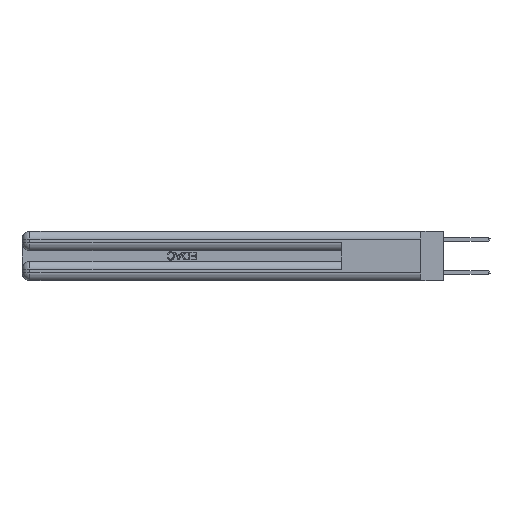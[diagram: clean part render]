
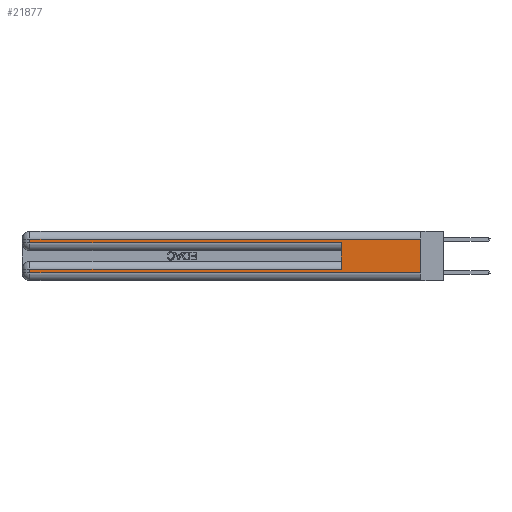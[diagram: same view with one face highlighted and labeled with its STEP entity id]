
A CAD part, left-side view. The second image highlights one B-rep face of the part: STEP entity #21877.
In plain terms, the highlighted planar face has unit normal (-1, 0, 0).
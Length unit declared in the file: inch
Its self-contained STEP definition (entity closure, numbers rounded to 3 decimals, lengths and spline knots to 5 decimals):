
#136 = PLANE ( 'NONE',  #1682 ) ;
#497 = DIRECTION ( 'NONE',  ( 0., -1., 0. ) ) ;
#635 = DIRECTION ( 'NONE',  ( 0., 0., -1. ) ) ;
#665 = VECTOR ( 'NONE', #23990, 39.37008 ) ;
#1326 = VECTOR ( 'NONE', #6034, 39.37008 ) ;
#1682 = AXIS2_PLACEMENT_3D ( 'NONE', #4948, #2603, #13789 ) ;
#1725 = CARTESIAN_POINT ( 'NONE',  ( 0., 0., 0.31 ) ) ;
#1740 = LINE ( 'NONE', #9009, #26144 ) ;
#2060 = CARTESIAN_POINT ( 'NONE',  ( 0., 2.94, 0.06 ) ) ;
#2248 = CARTESIAN_POINT ( 'NONE',  ( 0., 0.6, 0.085 ) ) ;
#2292 = DIRECTION ( 'NONE',  ( 0., 0., -1. ) ) ;
#2490 = ORIENTED_EDGE ( 'NONE', *, *, #18980, .T. ) ;
#2603 = DIRECTION ( 'NONE',  ( 1., 0., 0. ) ) ;
#2746 = CARTESIAN_POINT ( 'NONE',  ( 0., 2.94, 0.285 ) ) ;
#3892 = CARTESIAN_POINT ( 'NONE',  ( 0., 0., 0.06 ) ) ;
#4219 = VERTEX_POINT ( 'NONE', #11599 ) ;
#4916 = DIRECTION ( 'NONE',  ( 0., 0., -1. ) ) ;
#4948 = CARTESIAN_POINT ( 'NONE',  ( 0., 0., 0.37 ) ) ;
#5000 = CARTESIAN_POINT ( 'NONE',  ( 0., 2.94, 0.37 ) ) ;
#5064 = LINE ( 'NONE', #14529, #20643 ) ;
#6034 = DIRECTION ( 'NONE',  ( 0., 0., 1. ) ) ;
#6214 = CARTESIAN_POINT ( 'NONE',  ( 0., 0., 0.06 ) ) ;
#6603 = EDGE_LOOP ( 'NONE', ( #13898, #14363, #6667, #24856, #21002, #24072, #28019, #2490 ) ) ;
#6667 = ORIENTED_EDGE ( 'NONE', *, *, #11298, .T. ) ;
#7307 = VERTEX_POINT ( 'NONE', #20281 ) ;
#7476 = LINE ( 'NONE', #21756, #21827 ) ;
#7849 = VERTEX_POINT ( 'NONE', #2060 ) ;
#7964 = EDGE_CURVE ( 'NONE', #4219, #7849, #23902, .T. ) ;
#8282 = CARTESIAN_POINT ( 'NONE',  ( 0., 2.94, 0.31 ) ) ;
#8784 = EDGE_CURVE ( 'NONE', #11867, #4219, #19490, .T. ) ;
#9009 = CARTESIAN_POINT ( 'NONE',  ( 0., 0., 0.31 ) ) ;
#10094 = VECTOR ( 'NONE', #635, 39.37008 ) ;
#11298 = EDGE_CURVE ( 'NONE', #14647, #24955, #18730, .T. ) ;
#11599 = CARTESIAN_POINT ( 'NONE',  ( 0., 2.94, 0.085 ) ) ;
#11867 = VERTEX_POINT ( 'NONE', #2248 ) ;
#11905 = FACE_OUTER_BOUND ( 'NONE', #6603, .T. ) ;
#12609 = EDGE_CURVE ( 'NONE', #11867, #7307, #20307, .T. ) ;
#12863 = CARTESIAN_POINT ( 'NONE',  ( 0., 0.6, 0.145 ) ) ;
#13789 = DIRECTION ( 'NONE',  ( 0., 0., -1. ) ) ;
#13898 = ORIENTED_EDGE ( 'NONE', *, *, #25019, .F. ) ;
#13964 = VERTEX_POINT ( 'NONE', #1725 ) ;
#14363 = ORIENTED_EDGE ( 'NONE', *, *, #26984, .T. ) ;
#14529 = CARTESIAN_POINT ( 'NONE',  ( 0., 0., 0.37 ) ) ;
#14647 = VERTEX_POINT ( 'NONE', #8282 ) ;
#16368 = EDGE_CURVE ( 'NONE', #24955, #7307, #7476, .T. ) ;
#18730 = LINE ( 'NONE', #28023, #30343 ) ;
#18980 = EDGE_CURVE ( 'NONE', #7849, #20228, #20011, .T. ) ;
#19490 = LINE ( 'NONE', #26176, #665 ) ;
#20011 = LINE ( 'NONE', #3892, #27883 ) ;
#20228 = VERTEX_POINT ( 'NONE', #6214 ) ;
#20281 = CARTESIAN_POINT ( 'NONE',  ( 0., 0.6, 0.285 ) ) ;
#20307 = LINE ( 'NONE', #12863, #1326 ) ;
#20643 = VECTOR ( 'NONE', #2292, 39.37008 ) ;
#21002 = ORIENTED_EDGE ( 'NONE', *, *, #12609, .F. ) ;
#21756 = CARTESIAN_POINT ( 'NONE',  ( 0., 0., 0.285 ) ) ;
#21827 = VECTOR ( 'NONE', #497, 39.37008 ) ;
#21877 = ADVANCED_FACE ( 'NONE', ( #11905 ), #136, .F. ) ;
#22821 = DIRECTION ( 'NONE',  ( 0., 1., 0. ) ) ;
#23902 = LINE ( 'NONE', #5000, #10094 ) ;
#23990 = DIRECTION ( 'NONE',  ( 0., 1., 0. ) ) ;
#24072 = ORIENTED_EDGE ( 'NONE', *, *, #8784, .T. ) ;
#24856 = ORIENTED_EDGE ( 'NONE', *, *, #16368, .T. ) ;
#24955 = VERTEX_POINT ( 'NONE', #2746 ) ;
#25019 = EDGE_CURVE ( 'NONE', #13964, #20228, #5064, .T. ) ;
#26144 = VECTOR ( 'NONE', #22821, 39.37008 ) ;
#26176 = CARTESIAN_POINT ( 'NONE',  ( 0., 0., 0.085 ) ) ;
#26984 = EDGE_CURVE ( 'NONE', #13964, #14647, #1740, .T. ) ;
#27883 = VECTOR ( 'NONE', #29150, 39.37008 ) ;
#28019 = ORIENTED_EDGE ( 'NONE', *, *, #7964, .T. ) ;
#28023 = CARTESIAN_POINT ( 'NONE',  ( 0., 2.94, 0.37 ) ) ;
#29150 = DIRECTION ( 'NONE',  ( 0., -1., 0. ) ) ;
#30343 = VECTOR ( 'NONE', #4916, 39.37008 ) ;
